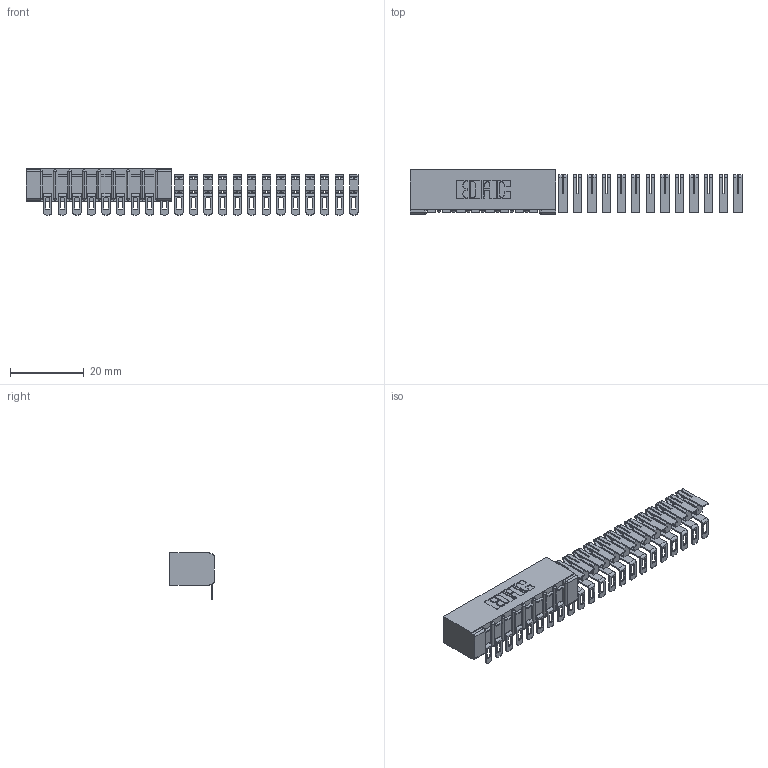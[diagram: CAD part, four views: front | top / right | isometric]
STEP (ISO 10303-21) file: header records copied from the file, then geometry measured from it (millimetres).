
FILE_DESCRIPTION (( 'STEP AP203' ), '1' );
FILE_NAME ('357-022-554-101.STEP', '2018-08-08T22:25:06', ( '' ), ( '' ), 'SwSTEP 2.0', 'SolidWorks 2016', '' );
FILE_SCHEMA (( 'CONFIG_CONTROL_DESIGN' ));
Length unit declared in the file: inch
Products named in the file (3): 307 Part_No Mounting Lugs; 307-290-002_554; 357-022-554-101
Assembly tree (23 placements, depth 2):
  357-022-554-101
    307 Part_No Mounting Lugs
    307-290-002_554  x22
Bounding box: 90.26 x 12.01 x 12.52 mm (x, y, z)
Volume: 3260.6 mm3; surface area: 8110.6 mm2
Topology: 23 solids, 23 shells, 1621 faces, 4969 edges, 3286 vertices
Faces by surface type: plane 910, cylinder 693, sphere 18
Entity records: 12185 total; most frequent: CARTESIAN_POINT 1988, DIRECTION 1966, ORIENTED_EDGE 1964, EDGE_CURVE 982, LINE 730, VECTOR 730, VERTEX_POINT 640, AXIS2_PLACEMENT_3D 618
